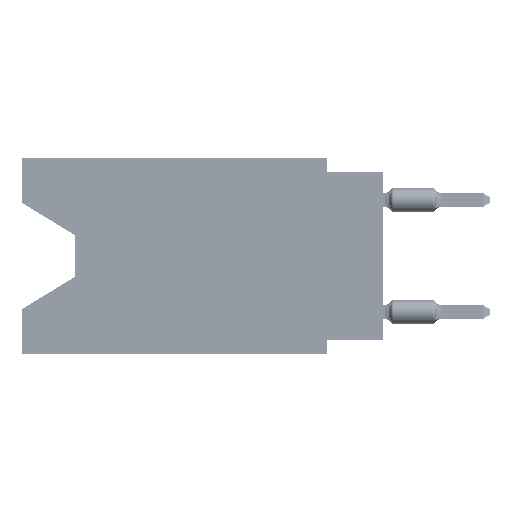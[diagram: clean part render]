
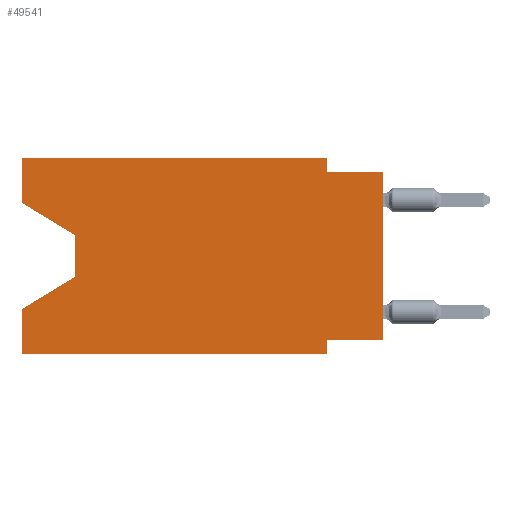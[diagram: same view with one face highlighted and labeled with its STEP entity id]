
A CAD part, left-side view. The second image highlights one B-rep face of the part: STEP entity #49541.
In plain terms, the highlighted planar face has unit normal (-1, 0, 0).
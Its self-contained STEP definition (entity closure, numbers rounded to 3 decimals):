
#4528 = CARTESIAN_POINT ( 'NONE',  ( 0., 16.383, -8.89 ) ) ;
#4859 = LINE ( 'NONE', #35358, #24859 ) ;
#4876 = VECTOR ( 'NONE', #70004, 1000. ) ;
#6463 = LINE ( 'NONE', #37355, #37630 ) ;
#8057 = VERTEX_POINT ( 'NONE', #23552 ) ;
#8219 = VERTEX_POINT ( 'NONE', #21447 ) ;
#8226 = CARTESIAN_POINT ( 'NONE',  ( 0., 2.54, 0. ) ) ;
#8689 = EDGE_CURVE ( 'NONE', #47656, #64126, #46539, .T. ) ;
#8912 = LINE ( 'NONE', #10106, #27176 ) ;
#9832 = ORIENTED_EDGE ( 'NONE', *, *, #70650, .T. ) ;
#10106 = CARTESIAN_POINT ( 'NONE',  ( 0., 13.97, -5.385 ) ) ;
#10668 = VERTEX_POINT ( 'NONE', #64918 ) ;
#11971 = CARTESIAN_POINT ( 'NONE',  ( 0., 0., 0. ) ) ;
#12352 = VERTEX_POINT ( 'NONE', #20979 ) ;
#13043 = CARTESIAN_POINT ( 'NONE',  ( 0., 13.97, -3.505 ) ) ;
#14309 = EDGE_CURVE ( 'NONE', #12352, #63436, #4859, .T. ) ;
#14368 = DIRECTION ( 'NONE',  ( 0., 1., 0. ) ) ;
#14467 = DIRECTION ( 'NONE',  ( 0., -1., 0. ) ) ;
#16616 = DIRECTION ( 'NONE',  ( 0., 0.855, -0.519 ) ) ;
#18124 = VERTEX_POINT ( 'NONE', #62300 ) ;
#18357 = DIRECTION ( 'NONE',  ( 0., 0., -1. ) ) ;
#19057 = DIRECTION ( 'NONE',  ( 0., 0., 1. ) ) ;
#19435 = ORIENTED_EDGE ( 'NONE', *, *, #69257, .F. ) ;
#19610 = DIRECTION ( 'NONE',  ( 0., 0., -1. ) ) ;
#19659 = DIRECTION ( 'NONE',  ( 0., 0., -1. ) ) ;
#20979 = CARTESIAN_POINT ( 'NONE',  ( 0., 0., -8.255 ) ) ;
#21186 = ORIENTED_EDGE ( 'NONE', *, *, #80179, .T. ) ;
#21218 = DIRECTION ( 'NONE',  ( 0., -1., 0. ) ) ;
#21447 = CARTESIAN_POINT ( 'NONE',  ( 0., 13.97, -5.385 ) ) ;
#22706 = LINE ( 'NONE', #58183, #24187 ) ;
#22894 = VECTOR ( 'NONE', #69074, 1000. ) ;
#23297 = LINE ( 'NONE', #48083, #22894 ) ;
#23552 = CARTESIAN_POINT ( 'NONE',  ( 0., 13.97, -3.505 ) ) ;
#23737 = ORIENTED_EDGE ( 'NONE', *, *, #8689, .F. ) ;
#23920 = ORIENTED_EDGE ( 'NONE', *, *, #46958, .F. ) ;
#24187 = VECTOR ( 'NONE', #21218, 1000. ) ;
#24346 = CARTESIAN_POINT ( 'NONE',  ( 0., 16.383, -2.038 ) ) ;
#24859 = VECTOR ( 'NONE', #14368, 1000. ) ;
#25034 = EDGE_CURVE ( 'NONE', #63436, #33579, #33047, .T. ) ;
#25540 = EDGE_CURVE ( 'NONE', #8219, #18124, #8912, .T. ) ;
#25871 = AXIS2_PLACEMENT_3D ( 'NONE', #50897, #31802, #19610 ) ;
#26025 = LINE ( 'NONE', #13043, #69716 ) ;
#27176 = VECTOR ( 'NONE', #16616, 1000. ) ;
#27865 = VERTEX_POINT ( 'NONE', #72105 ) ;
#29524 = DIRECTION ( 'NONE',  ( 0., 0., 1. ) ) ;
#30532 = VECTOR ( 'NONE', #29524, 1000. ) ;
#31802 = DIRECTION ( 'NONE',  ( 1., 0., 0. ) ) ;
#32164 = EDGE_LOOP ( 'NONE', ( #49380, #9832, #67022, #55572, #39769, #37439, #38693, #21186, #23737, #23920, #19435, #65148 ) ) ;
#32205 = PLANE ( 'NONE',  #25871 ) ;
#33047 = LINE ( 'NONE', #37940, #67561 ) ;
#33579 = VERTEX_POINT ( 'NONE', #70584 ) ;
#35358 = CARTESIAN_POINT ( 'NONE',  ( 0., 0., -8.255 ) ) ;
#35722 = CARTESIAN_POINT ( 'NONE',  ( 0., 2.54, -0.635 ) ) ;
#37355 = CARTESIAN_POINT ( 'NONE',  ( 0., 16.383, 0. ) ) ;
#37439 = ORIENTED_EDGE ( 'NONE', *, *, #25034, .F. ) ;
#37630 = VECTOR ( 'NONE', #19057, 1000. ) ;
#37940 = CARTESIAN_POINT ( 'NONE',  ( 0., 2.54, -8.89 ) ) ;
#38693 = ORIENTED_EDGE ( 'NONE', *, *, #14309, .F. ) ;
#39248 = CARTESIAN_POINT ( 'NONE',  ( 0., 0., -0.635 ) ) ;
#39769 = ORIENTED_EDGE ( 'NONE', *, *, #62938, .T. ) ;
#44479 = EDGE_CURVE ( 'NONE', #47163, #18124, #74220, .T. ) ;
#46539 = LINE ( 'NONE', #39248, #49228 ) ;
#46958 = EDGE_CURVE ( 'NONE', #52024, #47656, #50124, .T. ) ;
#47163 = VERTEX_POINT ( 'NONE', #4528 ) ;
#47656 = VERTEX_POINT ( 'NONE', #35722 ) ;
#48083 = CARTESIAN_POINT ( 'NONE',  ( 0., 16.383, -8.89 ) ) ;
#48470 = VECTOR ( 'NONE', #79423, 1000. ) ;
#49228 = VECTOR ( 'NONE', #14467, 1000. ) ;
#49380 = ORIENTED_EDGE ( 'NONE', *, *, #73116, .T. ) ;
#49541 = ADVANCED_FACE ( 'NONE', ( #75290 ), #32205, .F. ) ;
#49759 = LINE ( 'NONE', #11971, #48470 ) ;
#50124 = LINE ( 'NONE', #8226, #4876 ) ;
#50897 = CARTESIAN_POINT ( 'NONE',  ( 0., 16.383, 0. ) ) ;
#52024 = VERTEX_POINT ( 'NONE', #57114 ) ;
#55231 = LINE ( 'NONE', #24346, #60877 ) ;
#55572 = ORIENTED_EDGE ( 'NONE', *, *, #44479, .F. ) ;
#57114 = CARTESIAN_POINT ( 'NONE',  ( 0., 2.54, 0. ) ) ;
#58183 = CARTESIAN_POINT ( 'NONE',  ( 0., 16.383, 0. ) ) ;
#59881 = CARTESIAN_POINT ( 'NONE',  ( 0., 0., -0.635 ) ) ;
#60392 = CARTESIAN_POINT ( 'NONE',  ( 0., 16.383, 0. ) ) ;
#60877 = VECTOR ( 'NONE', #62117, 1000. ) ;
#61680 = CARTESIAN_POINT ( 'NONE',  ( 0., 2.54, -8.255 ) ) ;
#62117 = DIRECTION ( 'NONE',  ( 0., -0.855, -0.519 ) ) ;
#62300 = CARTESIAN_POINT ( 'NONE',  ( 0., 16.383, -6.852 ) ) ;
#62938 = EDGE_CURVE ( 'NONE', #47163, #33579, #23297, .T. ) ;
#63436 = VERTEX_POINT ( 'NONE', #61680 ) ;
#64126 = VERTEX_POINT ( 'NONE', #59881 ) ;
#64918 = CARTESIAN_POINT ( 'NONE',  ( 0., 16.383, 0. ) ) ;
#65148 = ORIENTED_EDGE ( 'NONE', *, *, #74373, .F. ) ;
#67022 = ORIENTED_EDGE ( 'NONE', *, *, #25540, .T. ) ;
#67561 = VECTOR ( 'NONE', #19659, 1000. ) ;
#69074 = DIRECTION ( 'NONE',  ( 0., -1., 0. ) ) ;
#69257 = EDGE_CURVE ( 'NONE', #10668, #52024, #22706, .T. ) ;
#69716 = VECTOR ( 'NONE', #18357, 1000. ) ;
#70004 = DIRECTION ( 'NONE',  ( 0., 0., -1. ) ) ;
#70584 = CARTESIAN_POINT ( 'NONE',  ( 0., 2.54, -8.89 ) ) ;
#70650 = EDGE_CURVE ( 'NONE', #8057, #8219, #26025, .T. ) ;
#72105 = CARTESIAN_POINT ( 'NONE',  ( 0., 16.383, -2.038 ) ) ;
#73116 = EDGE_CURVE ( 'NONE', #27865, #8057, #55231, .T. ) ;
#74220 = LINE ( 'NONE', #60392, #30532 ) ;
#74373 = EDGE_CURVE ( 'NONE', #27865, #10668, #6463, .T. ) ;
#75290 = FACE_OUTER_BOUND ( 'NONE', #32164, .T. ) ;
#79423 = DIRECTION ( 'NONE',  ( 0., 0., 1. ) ) ;
#80179 = EDGE_CURVE ( 'NONE', #12352, #64126, #49759, .T. ) ;
